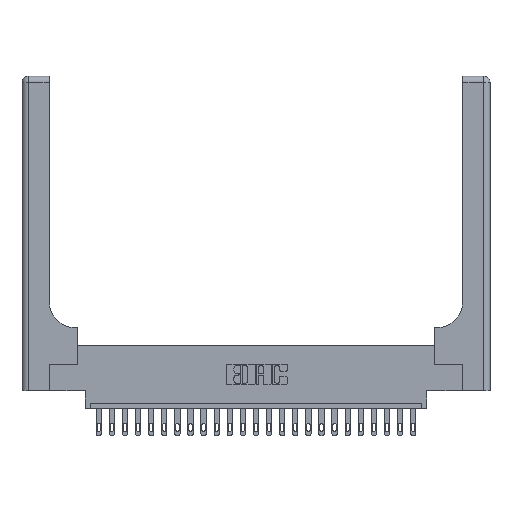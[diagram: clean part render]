
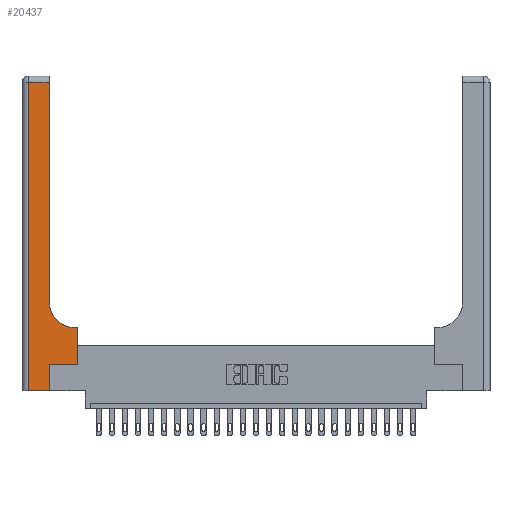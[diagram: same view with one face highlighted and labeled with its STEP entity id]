
A CAD part, top view. The second image highlights one B-rep face of the part: STEP entity #20437.
In plain terms, the highlighted planar face has unit normal (0, 0, 1).
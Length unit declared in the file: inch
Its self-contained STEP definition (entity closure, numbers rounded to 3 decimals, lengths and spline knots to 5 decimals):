
#383 = AXIS2_PLACEMENT_3D ( 'NONE', #10317, #11637, #17604 ) ;
#557 = EDGE_CURVE ( 'NONE', #19667, #8325, #3024, .T. ) ;
#871 = ORIENTED_EDGE ( 'NONE', *, *, #557, .T. ) ;
#1204 = LINE ( 'NONE', #5028, #5369 ) ;
#2322 = VECTOR ( 'NONE', #14389, 39.37008 ) ;
#2660 = DIRECTION ( 'NONE',  ( 0., 1., 0. ) ) ;
#3024 = LINE ( 'NONE', #10255, #17732 ) ;
#3167 = CARTESIAN_POINT ( 'NONE',  ( 0.26, 2.94, 0.37 ) ) ;
#3328 = EDGE_CURVE ( 'NONE', #5811, #19667, #5712, .T. ) ;
#3397 = ORIENTED_EDGE ( 'NONE', *, *, #23302, .T. ) ;
#4471 = ORIENTED_EDGE ( 'NONE', *, *, #12457, .T. ) ;
#4567 = LINE ( 'NONE', #22871, #23213 ) ;
#5028 = CARTESIAN_POINT ( 'NONE',  ( 0.26, 3., 0.37 ) ) ;
#5087 = EDGE_CURVE ( 'NONE', #15061, #14592, #23413, .T. ) ;
#5226 = PLANE ( 'NONE',  #22724 ) ;
#5305 = CARTESIAN_POINT ( 'NONE',  ( 0.26, 0.6, 0.37 ) ) ;
#5342 = DIRECTION ( 'NONE',  ( 0., 0., -1. ) ) ;
#5369 = VECTOR ( 'NONE', #21328, 39.37008 ) ;
#5712 = LINE ( 'NONE', #7478, #11744 ) ;
#5811 = VERTEX_POINT ( 'NONE', #14119 ) ;
#5920 = CARTESIAN_POINT ( 'NONE',  ( 0.528, 0.25, 0.37 ) ) ;
#5983 = CARTESIAN_POINT ( 'NONE',  ( 0.528, 0.6, 0.37 ) ) ;
#6536 = CARTESIAN_POINT ( 'NONE',  ( 0.265, 0.25, 0.37 ) ) ;
#6629 = EDGE_CURVE ( 'NONE', #23311, #23068, #1204, .T. ) ;
#7002 = DIRECTION ( 'NONE',  ( -1., 0., 0. ) ) ;
#7124 = CARTESIAN_POINT ( 'NONE',  ( 0.528, 0.25, 0.37 ) ) ;
#7478 = CARTESIAN_POINT ( 'NONE',  ( 0.06, 3., 0.37 ) ) ;
#7669 = ORIENTED_EDGE ( 'NONE', *, *, #6629, .T. ) ;
#8325 = VERTEX_POINT ( 'NONE', #22700 ) ;
#8486 = DIRECTION ( 'NONE',  ( 1., 0., 0. ) ) ;
#8964 = LINE ( 'NONE', #14464, #20551 ) ;
#9001 = VECTOR ( 'NONE', #15844, 39.37008 ) ;
#9919 = ORIENTED_EDGE ( 'NONE', *, *, #18702, .T. ) ;
#10255 = CARTESIAN_POINT ( 'NONE',  ( 0., 0., 0.37 ) ) ;
#10317 = CARTESIAN_POINT ( 'NONE',  ( 0.51, 0.85, 0.37 ) ) ;
#10341 = LINE ( 'NONE', #17625, #9001 ) ;
#10554 = CARTESIAN_POINT ( 'NONE',  ( 0., 3., 0.37 ) ) ;
#11637 = DIRECTION ( 'NONE',  ( 0., 0., -1. ) ) ;
#11744 = VECTOR ( 'NONE', #19886, 39.37008 ) ;
#12188 = VECTOR ( 'NONE', #18036, 39.37008 ) ;
#12282 = EDGE_LOOP ( 'NONE', ( #7669, #19368, #14767, #871, #3397, #9919, #19078, #18120, #4471 ) ) ;
#12457 = EDGE_CURVE ( 'NONE', #18980, #23311, #22762, .T. ) ;
#13511 = VERTEX_POINT ( 'NONE', #6536 ) ;
#13725 = CARTESIAN_POINT ( 'NONE',  ( 0.26, 0.85, 0.37 ) ) ;
#13997 = CARTESIAN_POINT ( 'NONE',  ( 0.06, 0., 0.37 ) ) ;
#14119 = CARTESIAN_POINT ( 'NONE',  ( 0.06, 2.94, 0.37 ) ) ;
#14389 = DIRECTION ( 'NONE',  ( 0., 1., 0. ) ) ;
#14464 = CARTESIAN_POINT ( 'NONE',  ( 0., 2.94, 0.37 ) ) ;
#14592 = VERTEX_POINT ( 'NONE', #5983 ) ;
#14767 = ORIENTED_EDGE ( 'NONE', *, *, #3328, .T. ) ;
#15061 = VERTEX_POINT ( 'NONE', #5920 ) ;
#15221 = CARTESIAN_POINT ( 'NONE',  ( 0.51, 0.6, 0.37 ) ) ;
#15844 = DIRECTION ( 'NONE',  ( 1., 0., 0. ) ) ;
#17604 = DIRECTION ( 'NONE',  ( 1., 0., 0. ) ) ;
#17625 = CARTESIAN_POINT ( 'NONE',  ( 0.265, 0.25, 0.37 ) ) ;
#17732 = VECTOR ( 'NONE', #8486, 39.37008 ) ;
#18036 = DIRECTION ( 'NONE',  ( -1., 0., 0. ) ) ;
#18120 = ORIENTED_EDGE ( 'NONE', *, *, #22972, .T. ) ;
#18702 = EDGE_CURVE ( 'NONE', #13511, #15061, #10341, .T. ) ;
#18980 = VERTEX_POINT ( 'NONE', #15221 ) ;
#19078 = ORIENTED_EDGE ( 'NONE', *, *, #5087, .T. ) ;
#19368 = ORIENTED_EDGE ( 'NONE', *, *, #23008, .T. ) ;
#19470 = LINE ( 'NONE', #5305, #12188 ) ;
#19667 = VERTEX_POINT ( 'NONE', #13997 ) ;
#19886 = DIRECTION ( 'NONE',  ( 0., -1., 0. ) ) ;
#19932 = DIRECTION ( 'NONE',  ( -1., 0., 0. ) ) ;
#20437 = ADVANCED_FACE ( 'NONE', ( #23055 ), #5226, .F. ) ;
#20551 = VECTOR ( 'NONE', #19932, 39.37008 ) ;
#21328 = DIRECTION ( 'NONE',  ( 0., 1., 0. ) ) ;
#22700 = CARTESIAN_POINT ( 'NONE',  ( 0.265, 0., 0.37 ) ) ;
#22724 = AXIS2_PLACEMENT_3D ( 'NONE', #10554, #5342, #7002 ) ;
#22762 = CIRCLE ( 'NONE', #383, 0.25 ) ;
#22871 = CARTESIAN_POINT ( 'NONE',  ( 0.265, 0., 0.37 ) ) ;
#22972 = EDGE_CURVE ( 'NONE', #14592, #18980, #19470, .T. ) ;
#23008 = EDGE_CURVE ( 'NONE', #23068, #5811, #8964, .T. ) ;
#23055 = FACE_OUTER_BOUND ( 'NONE', #12282, .T. ) ;
#23068 = VERTEX_POINT ( 'NONE', #3167 ) ;
#23213 = VECTOR ( 'NONE', #2660, 39.37008 ) ;
#23302 = EDGE_CURVE ( 'NONE', #8325, #13511, #4567, .T. ) ;
#23311 = VERTEX_POINT ( 'NONE', #13725 ) ;
#23413 = LINE ( 'NONE', #7124, #2322 ) ;
